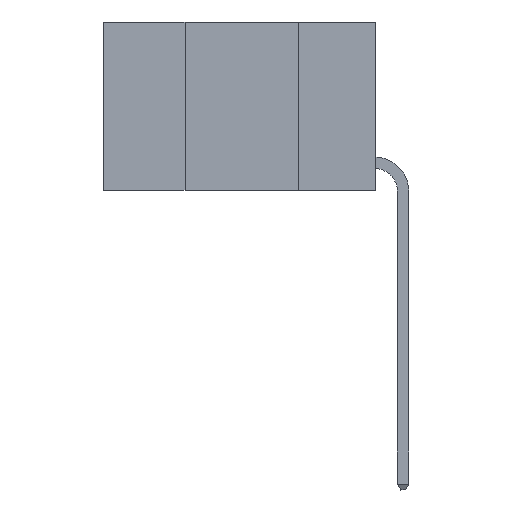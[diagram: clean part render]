
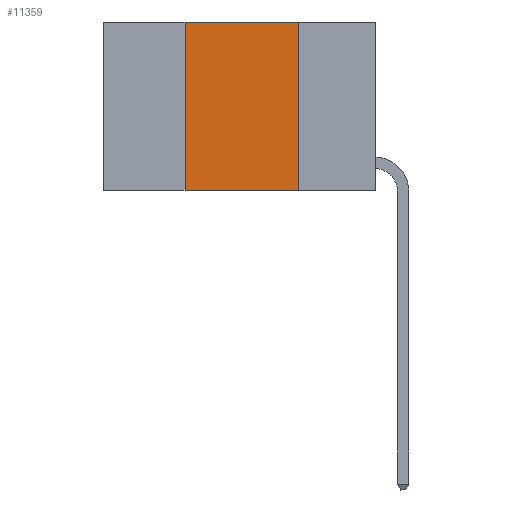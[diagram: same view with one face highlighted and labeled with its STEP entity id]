
A CAD part, left-side view. The second image highlights one B-rep face of the part: STEP entity #11359.
In plain terms, the highlighted planar face has unit normal (-1, 0, 0).
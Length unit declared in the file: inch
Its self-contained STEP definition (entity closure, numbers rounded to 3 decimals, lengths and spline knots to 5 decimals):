
#86 = CARTESIAN_POINT ( 'NONE',  ( 0., 0.17, -0.37 ) ) ;
#1265 = FACE_OUTER_BOUND ( 'NONE', #10238, .T. ) ;
#1880 = DIRECTION ( 'NONE',  ( 0., -1., 0. ) ) ;
#1956 = CARTESIAN_POINT ( 'NONE',  ( 0., 0.6, -0.37 ) ) ;
#2245 = VECTOR ( 'NONE', #5975, 39.37008 ) ;
#2288 = EDGE_CURVE ( 'NONE', #2489, #12417, #14713, .T. ) ;
#2489 = VERTEX_POINT ( 'NONE', #3823 ) ;
#3035 = VERTEX_POINT ( 'NONE', #86 ) ;
#3823 = CARTESIAN_POINT ( 'NONE',  ( 0., 0.42, -0.37 ) ) ;
#4380 = PLANE ( 'NONE',  #14745 ) ;
#4704 = CARTESIAN_POINT ( 'NONE',  ( 0., 0.6, 0. ) ) ;
#5502 = CARTESIAN_POINT ( 'NONE',  ( 0., 0.6, 0. ) ) ;
#5975 = DIRECTION ( 'NONE',  ( 0., -1., 0. ) ) ;
#6379 = CARTESIAN_POINT ( 'NONE',  ( 0., 0.17, 0. ) ) ;
#6894 = DIRECTION ( 'NONE',  ( 0., 0., -1. ) ) ;
#7473 = DIRECTION ( 'NONE',  ( 0., 0., 1. ) ) ;
#8057 = ORIENTED_EDGE ( 'NONE', *, *, #2288, .F. ) ;
#8951 = LINE ( 'NONE', #1956, #2245 ) ;
#9063 = LINE ( 'NONE', #4704, #17447 ) ;
#9347 = VECTOR ( 'NONE', #7473, 39.37008 ) ;
#9628 = EDGE_CURVE ( 'NONE', #11862, #3035, #16287, .T. ) ;
#10238 = EDGE_LOOP ( 'NONE', ( #15686, #11783, #8057, #16808 ) ) ;
#10597 = CARTESIAN_POINT ( 'NONE',  ( 0., 0.17, 0. ) ) ;
#10642 = EDGE_CURVE ( 'NONE', #12417, #11862, #9063, .T. ) ;
#11057 = EDGE_CURVE ( 'NONE', #2489, #3035, #8951, .T. ) ;
#11068 = DIRECTION ( 'NONE',  ( 1., 0., 0. ) ) ;
#11359 = ADVANCED_FACE ( 'NONE', ( #1265 ), #4380, .F. ) ;
#11783 = ORIENTED_EDGE ( 'NONE', *, *, #10642, .F. ) ;
#11862 = VERTEX_POINT ( 'NONE', #6379 ) ;
#12079 = DIRECTION ( 'NONE',  ( 0., 0., -1. ) ) ;
#12417 = VERTEX_POINT ( 'NONE', #14095 ) ;
#13506 = CARTESIAN_POINT ( 'NONE',  ( 0., 0.42, 0. ) ) ;
#14095 = CARTESIAN_POINT ( 'NONE',  ( 0., 0.42, 0. ) ) ;
#14713 = LINE ( 'NONE', #13506, #9347 ) ;
#14745 = AXIS2_PLACEMENT_3D ( 'NONE', #5502, #11068, #6894 ) ;
#15686 = ORIENTED_EDGE ( 'NONE', *, *, #9628, .F. ) ;
#16287 = LINE ( 'NONE', #10597, #18300 ) ;
#16808 = ORIENTED_EDGE ( 'NONE', *, *, #11057, .T. ) ;
#17447 = VECTOR ( 'NONE', #1880, 39.37008 ) ;
#18300 = VECTOR ( 'NONE', #12079, 39.37008 ) ;
